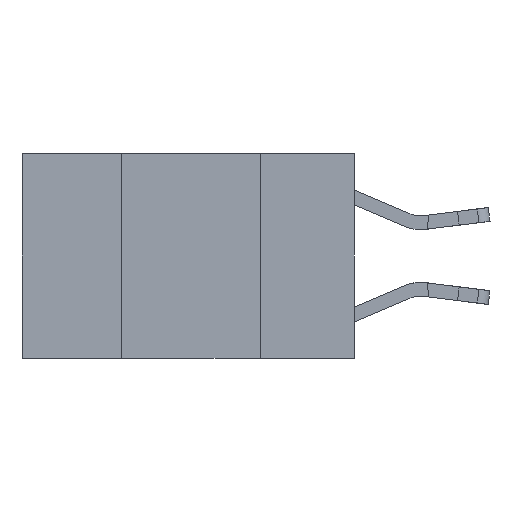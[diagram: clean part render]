
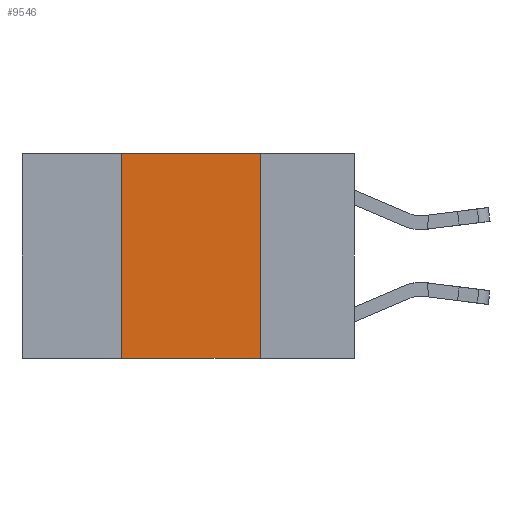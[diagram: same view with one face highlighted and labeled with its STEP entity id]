
A CAD part, left-side view. The second image highlights one B-rep face of the part: STEP entity #9546.
In plain terms, the highlighted planar face has unit normal (-1, 0, 0).
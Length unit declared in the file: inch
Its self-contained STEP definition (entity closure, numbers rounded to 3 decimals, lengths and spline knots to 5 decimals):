
#558 = VECTOR ( 'NONE', #7679, 39.37008 ) ;
#616 = EDGE_CURVE ( 'NONE', #7515, #13015, #10265, .T. ) ;
#763 = DIRECTION ( 'NONE',  ( 1., 0., 0. ) ) ;
#1286 = ORIENTED_EDGE ( 'NONE', *, *, #16471, .F. ) ;
#1389 = LINE ( 'NONE', #7899, #558 ) ;
#1908 = CARTESIAN_POINT ( 'NONE',  ( 0., 0.42, 0. ) ) ;
#1988 = VECTOR ( 'NONE', #14257, 39.37008 ) ;
#2263 = EDGE_CURVE ( 'NONE', #10874, #7515, #1389, .T. ) ;
#2806 = LINE ( 'NONE', #5223, #1988 ) ;
#3453 = VECTOR ( 'NONE', #4574, 39.37008 ) ;
#4424 = CARTESIAN_POINT ( 'NONE',  ( 0., 0.42, 0. ) ) ;
#4574 = DIRECTION ( 'NONE',  ( 0., 0., -1. ) ) ;
#4575 = PLANE ( 'NONE',  #7211 ) ;
#4651 = EDGE_LOOP ( 'NONE', ( #14180, #11119, #1286, #5081 ) ) ;
#5081 = ORIENTED_EDGE ( 'NONE', *, *, #15616, .T. ) ;
#5223 = CARTESIAN_POINT ( 'NONE',  ( 0., 0.6, -0.37 ) ) ;
#7211 = AXIS2_PLACEMENT_3D ( 'NONE', #8453, #763, #9742 ) ;
#7515 = VERTEX_POINT ( 'NONE', #15760 ) ;
#7679 = DIRECTION ( 'NONE',  ( 0., -1., 0. ) ) ;
#7899 = CARTESIAN_POINT ( 'NONE',  ( 0., 0.6, 0. ) ) ;
#8453 = CARTESIAN_POINT ( 'NONE',  ( 0., 0.6, 0. ) ) ;
#9177 = LINE ( 'NONE', #1908, #9567 ) ;
#9295 = VERTEX_POINT ( 'NONE', #10480 ) ;
#9546 = ADVANCED_FACE ( 'NONE', ( #15734 ), #4575, .F. ) ;
#9567 = VECTOR ( 'NONE', #12195, 39.37008 ) ;
#9742 = DIRECTION ( 'NONE',  ( 0., 0., -1. ) ) ;
#10265 = LINE ( 'NONE', #14612, #3453 ) ;
#10480 = CARTESIAN_POINT ( 'NONE',  ( 0., 0.42, -0.37 ) ) ;
#10874 = VERTEX_POINT ( 'NONE', #4424 ) ;
#11119 = ORIENTED_EDGE ( 'NONE', *, *, #2263, .F. ) ;
#12195 = DIRECTION ( 'NONE',  ( 0., 0., 1. ) ) ;
#12783 = CARTESIAN_POINT ( 'NONE',  ( 0., 0.17, -0.37 ) ) ;
#13015 = VERTEX_POINT ( 'NONE', #12783 ) ;
#14180 = ORIENTED_EDGE ( 'NONE', *, *, #616, .F. ) ;
#14257 = DIRECTION ( 'NONE',  ( 0., -1., 0. ) ) ;
#14612 = CARTESIAN_POINT ( 'NONE',  ( 0., 0.17, 0. ) ) ;
#15616 = EDGE_CURVE ( 'NONE', #9295, #13015, #2806, .T. ) ;
#15734 = FACE_OUTER_BOUND ( 'NONE', #4651, .T. ) ;
#15760 = CARTESIAN_POINT ( 'NONE',  ( 0., 0.17, 0. ) ) ;
#16471 = EDGE_CURVE ( 'NONE', #9295, #10874, #9177, .T. ) ;
